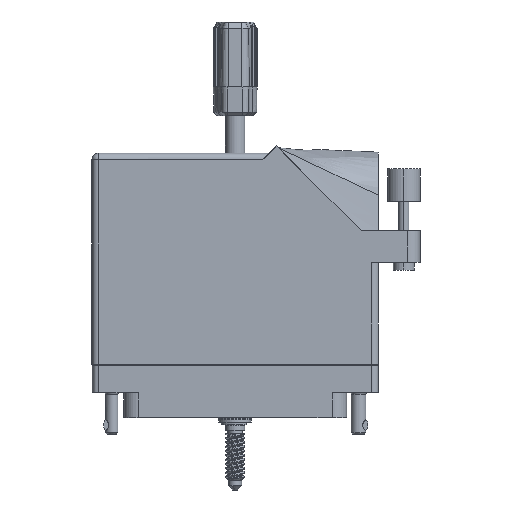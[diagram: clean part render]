
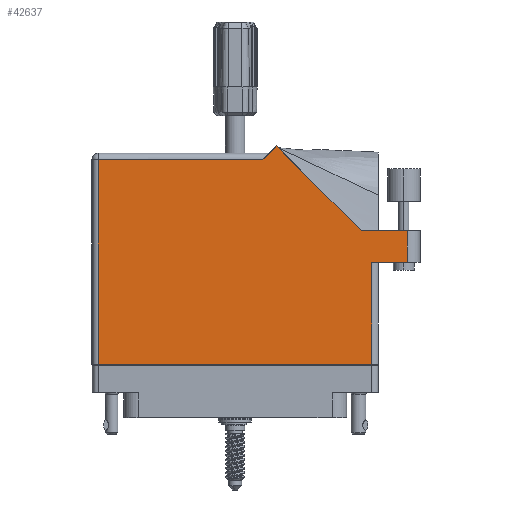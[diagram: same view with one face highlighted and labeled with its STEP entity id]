
A CAD part, front view. The second image highlights one B-rep face of the part: STEP entity #42637.
In plain terms, the highlighted face is planar.
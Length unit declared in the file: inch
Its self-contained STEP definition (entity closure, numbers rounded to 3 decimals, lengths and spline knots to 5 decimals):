
#6024 = EDGE_CURVE ( 'NONE', #108159, #40584, #87370, .T. ) ;
#6596 = LINE ( 'NONE', #12025, #71315 ) ;
#7867 = ORIENTED_EDGE ( 'NONE', *, *, #42863, .T. ) ;
#10133 = VERTEX_POINT ( 'NONE', #88953 ) ;
#10192 = DIRECTION ( 'NONE',  ( -1., 0., 0. ) ) ;
#10594 = DIRECTION ( 'NONE',  ( 0., -1., 0. ) ) ;
#11789 = VECTOR ( 'NONE', #24264, 39.37008 ) ;
#12025 = CARTESIAN_POINT ( 'NONE',  ( -1.3155, -0.1, 0.765 ) ) ;
#14008 = ORIENTED_EDGE ( 'NONE', *, *, #87905, .T. ) ;
#20656 = VECTOR ( 'NONE', #33649, 39.37008 ) ;
#22214 = DIRECTION ( 'NONE',  ( 1., 0., 0. ) ) ;
#24264 = DIRECTION ( 'NONE',  ( -1., 0., 0. ) ) ;
#25043 = VECTOR ( 'NONE', #49781, 39.37008 ) ;
#25060 = VERTEX_POINT ( 'NONE', #29754 ) ;
#25465 = CARTESIAN_POINT ( 'NONE',  ( -1.3775, -0.1, 0.765 ) ) ;
#25791 = CARTESIAN_POINT ( 'NONE',  ( -1.3775, 1.868, 0.765 ) ) ;
#26768 = FACE_OUTER_BOUND ( 'NONE', #30360, .T. ) ;
#27476 = CARTESIAN_POINT ( 'NONE',  ( -1.3775, 1.93, 0.765 ) ) ;
#28426 = ORIENTED_EDGE ( 'NONE', *, *, #73875, .T. ) ;
#28438 = VECTOR ( 'NONE', #84693, 39.37008 ) ;
#29754 = CARTESIAN_POINT ( 'NONE',  ( 1.3155, 0.88, 0.765 ) ) ;
#30276 = CARTESIAN_POINT ( 'NONE',  ( 1.6525, 1.187, 0.765 ) ) ;
#30360 = EDGE_LOOP ( 'NONE', ( #98644, #60515, #14008, #68816, #41675, #7867, #51261, #79175, #28426 ) ) ;
#31225 = LINE ( 'NONE', #78732, #73533 ) ;
#33033 = LINE ( 'NONE', #55345, #25043 ) ;
#33606 = DIRECTION ( 'NONE',  ( -1., 0., 0. ) ) ;
#33649 = DIRECTION ( 'NONE',  ( 1., 0., 0. ) ) ;
#34216 = EDGE_CURVE ( 'NONE', #53313, #108159, #58285, .T. ) ;
#36529 = CARTESIAN_POINT ( 'NONE',  ( -1.3155, -0.1, 0.765 ) ) ;
#37275 = CARTESIAN_POINT ( 'NONE',  ( -1.3155, 1.868, 0.765 ) ) ;
#40584 = VERTEX_POINT ( 'NONE', #81292 ) ;
#40898 = CARTESIAN_POINT ( 'NONE',  ( 1.7775, 1.187, 0.765 ) ) ;
#41675 = ORIENTED_EDGE ( 'NONE', *, *, #6024, .T. ) ;
#42637 = ADVANCED_FACE ( 'NONE', ( #26768 ), #60803, .F. ) ;
#42863 = EDGE_CURVE ( 'NONE', #40584, #76370, #88023, .T. ) ;
#43142 = LINE ( 'NONE', #25465, #20656 ) ;
#47378 = CARTESIAN_POINT ( 'NONE',  ( 0.3275, 1.93, 0.765 ) ) ;
#49781 = DIRECTION ( 'NONE',  ( 0., 1., 0. ) ) ;
#50191 = LINE ( 'NONE', #40898, #11789 ) ;
#50745 = CARTESIAN_POINT ( 'NONE',  ( 1.3155, 0.88, 0.765 ) ) ;
#51261 = ORIENTED_EDGE ( 'NONE', *, *, #82276, .T. ) ;
#51911 = DIRECTION ( 'NONE',  ( 0., 0., -1. ) ) ;
#53313 = VERTEX_POINT ( 'NONE', #68696 ) ;
#54434 = CARTESIAN_POINT ( 'NONE',  ( 1.21192, 1.187, 0.765 ) ) ;
#55345 = CARTESIAN_POINT ( 'NONE',  ( 1.6525, 1.187, 0.765 ) ) ;
#56894 = VECTOR ( 'NONE', #62193, 39.37008 ) ;
#58285 = LINE ( 'NONE', #54434, #56894 ) ;
#60515 = ORIENTED_EDGE ( 'NONE', *, *, #64215, .T. ) ;
#60803 = PLANE ( 'NONE',  #88157 ) ;
#62193 = DIRECTION ( 'NONE',  ( -0.707, 0.707, 0. ) ) ;
#64215 = EDGE_CURVE ( 'NONE', #10133, #65380, #33033, .T. ) ;
#65380 = VERTEX_POINT ( 'NONE', #30276 ) ;
#68696 = CARTESIAN_POINT ( 'NONE',  ( 1.21192, 1.187, 0.765 ) ) ;
#68816 = ORIENTED_EDGE ( 'NONE', *, *, #34216, .T. ) ;
#70250 = VECTOR ( 'NONE', #80592, 39.37008 ) ;
#71315 = VECTOR ( 'NONE', #10594, 39.37008 ) ;
#73533 = VECTOR ( 'NONE', #22214, 39.37008 ) ;
#73875 = EDGE_CURVE ( 'NONE', #77855, #25060, #76064, .T. ) ;
#76064 = LINE ( 'NONE', #50745, #28438 ) ;
#76370 = VERTEX_POINT ( 'NONE', #37275 ) ;
#76868 = CARTESIAN_POINT ( 'NONE',  ( 1.3155, -0.1, 0.765 ) ) ;
#77855 = VERTEX_POINT ( 'NONE', #76868 ) ;
#78732 = CARTESIAN_POINT ( 'NONE',  ( 1.3775, 0.88, 0.765 ) ) ;
#79175 = ORIENTED_EDGE ( 'NONE', *, *, #85043, .T. ) ;
#80592 = DIRECTION ( 'NONE',  ( -0.707, -0.707, 0. ) ) ;
#81292 = CARTESIAN_POINT ( 'NONE',  ( 0.2655, 1.868, 0.765 ) ) ;
#82276 = EDGE_CURVE ( 'NONE', #76370, #85349, #6596, .T. ) ;
#84693 = DIRECTION ( 'NONE',  ( 0., 1., 0. ) ) ;
#84826 = EDGE_CURVE ( 'NONE', #25060, #10133, #31225, .T. ) ;
#85043 = EDGE_CURVE ( 'NONE', #85349, #77855, #43142, .T. ) ;
#85349 = VERTEX_POINT ( 'NONE', #36529 ) ;
#85787 = CARTESIAN_POINT ( 'NONE',  ( 0.39821, 2.00071, 0.765 ) ) ;
#87370 = LINE ( 'NONE', #47378, #70250 ) ;
#87905 = EDGE_CURVE ( 'NONE', #65380, #53313, #50191, .T. ) ;
#88023 = LINE ( 'NONE', #25791, #93200 ) ;
#88157 = AXIS2_PLACEMENT_3D ( 'NONE', #27476, #51911, #10192 ) ;
#88953 = CARTESIAN_POINT ( 'NONE',  ( 1.6525, 0.88, 0.765 ) ) ;
#93200 = VECTOR ( 'NONE', #33606, 39.37008 ) ;
#98644 = ORIENTED_EDGE ( 'NONE', *, *, #84826, .T. ) ;
#108159 = VERTEX_POINT ( 'NONE', #85787 ) ;
